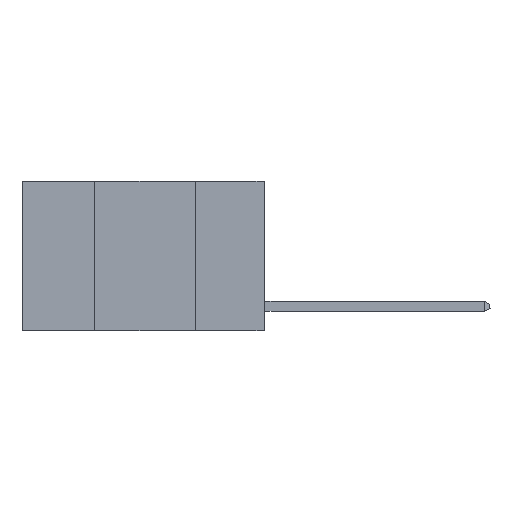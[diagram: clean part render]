
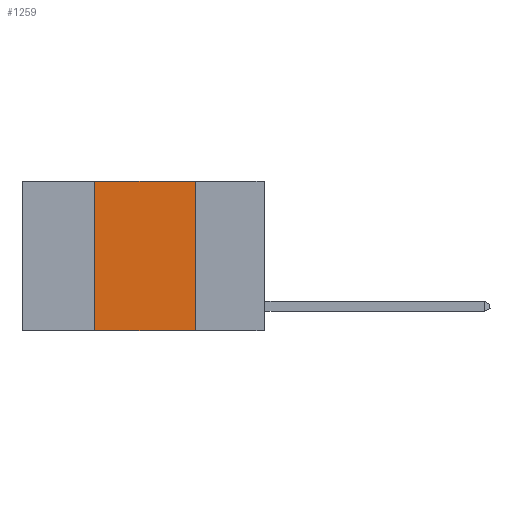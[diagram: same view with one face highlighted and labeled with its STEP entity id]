
A CAD part, left-side view. The second image highlights one B-rep face of the part: STEP entity #1259.
In plain terms, the highlighted planar face has unit normal (-1, 0, 0).
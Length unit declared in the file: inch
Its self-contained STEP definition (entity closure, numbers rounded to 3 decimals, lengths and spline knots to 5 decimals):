
#134 = AXIS2_PLACEMENT_3D ( 'NONE', #9417, #9370, #4114 ) ;
#581 = CARTESIAN_POINT ( 'NONE',  ( 0., 0.17, 0. ) ) ;
#586 = EDGE_LOOP ( 'NONE', ( #9858, #8731, #8334, #8155 ) ) ;
#709 = CARTESIAN_POINT ( 'NONE',  ( 0., 0.42, 0. ) ) ;
#890 = EDGE_CURVE ( 'NONE', #5016, #4737, #6654, .T. ) ;
#1259 = ADVANCED_FACE ( 'NONE', ( #5491 ), #8612, .F. ) ;
#1989 = VECTOR ( 'NONE', #3732, 39.37008 ) ;
#2028 = CARTESIAN_POINT ( 'NONE',  ( 0., 0.42, -0.37 ) ) ;
#2611 = VECTOR ( 'NONE', #7708, 39.37008 ) ;
#3422 = VERTEX_POINT ( 'NONE', #8516 ) ;
#3732 = DIRECTION ( 'NONE',  ( 0., 0., -1. ) ) ;
#4114 = DIRECTION ( 'NONE',  ( 0., 0., -1. ) ) ;
#4600 = LINE ( 'NONE', #709, #6900 ) ;
#4737 = VERTEX_POINT ( 'NONE', #7556 ) ;
#4789 = VERTEX_POINT ( 'NONE', #5423 ) ;
#5016 = VERTEX_POINT ( 'NONE', #2028 ) ;
#5336 = LINE ( 'NONE', #9779, #2611 ) ;
#5423 = CARTESIAN_POINT ( 'NONE',  ( 0., 0.17, 0. ) ) ;
#5491 = FACE_OUTER_BOUND ( 'NONE', #586, .T. ) ;
#6578 = EDGE_CURVE ( 'NONE', #3422, #4789, #5336, .T. ) ;
#6654 = LINE ( 'NONE', #7554, #6902 ) ;
#6686 = LINE ( 'NONE', #581, #1989 ) ;
#6900 = VECTOR ( 'NONE', #7650, 39.37008 ) ;
#6902 = VECTOR ( 'NONE', #8918, 39.37008 ) ;
#7554 = CARTESIAN_POINT ( 'NONE',  ( 0., 0.6, -0.37 ) ) ;
#7556 = CARTESIAN_POINT ( 'NONE',  ( 0., 0.17, -0.37 ) ) ;
#7650 = DIRECTION ( 'NONE',  ( 0., 0., 1. ) ) ;
#7708 = DIRECTION ( 'NONE',  ( 0., -1., 0. ) ) ;
#8155 = ORIENTED_EDGE ( 'NONE', *, *, #890, .T. ) ;
#8334 = ORIENTED_EDGE ( 'NONE', *, *, #9512, .F. ) ;
#8516 = CARTESIAN_POINT ( 'NONE',  ( 0., 0.42, 0. ) ) ;
#8612 = PLANE ( 'NONE',  #134 ) ;
#8731 = ORIENTED_EDGE ( 'NONE', *, *, #6578, .F. ) ;
#8754 = EDGE_CURVE ( 'NONE', #4789, #4737, #6686, .T. ) ;
#8918 = DIRECTION ( 'NONE',  ( 0., -1., 0. ) ) ;
#9370 = DIRECTION ( 'NONE',  ( 1., 0., 0. ) ) ;
#9417 = CARTESIAN_POINT ( 'NONE',  ( 0., 0.6, 0. ) ) ;
#9512 = EDGE_CURVE ( 'NONE', #5016, #3422, #4600, .T. ) ;
#9779 = CARTESIAN_POINT ( 'NONE',  ( 0., 0.6, 0. ) ) ;
#9858 = ORIENTED_EDGE ( 'NONE', *, *, #8754, .F. ) ;
